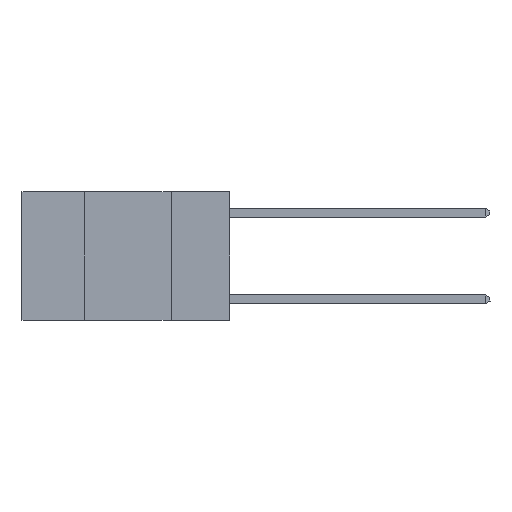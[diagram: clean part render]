
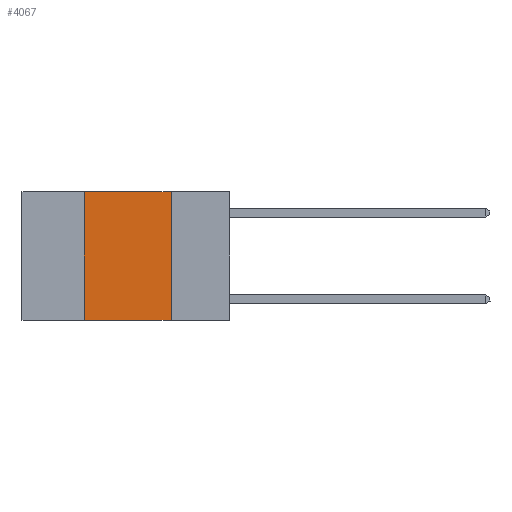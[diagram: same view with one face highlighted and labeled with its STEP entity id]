
A CAD part, left-side view. The second image highlights one B-rep face of the part: STEP entity #4067.
In plain terms, the highlighted planar face has unit normal (-1, 0, 0).
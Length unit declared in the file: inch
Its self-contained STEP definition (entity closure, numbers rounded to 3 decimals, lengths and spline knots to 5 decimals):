
#283 = DIRECTION ( 'NONE',  ( 0., 0., 1. ) ) ;
#315 = ORIENTED_EDGE ( 'NONE', *, *, #3388, .T. ) ;
#1028 = VERTEX_POINT ( 'NONE', #6104 ) ;
#1468 = EDGE_CURVE ( 'NONE', #9385, #1028, #7223, .T. ) ;
#1759 = CARTESIAN_POINT ( 'NONE',  ( 0., 0.42, 0. ) ) ;
#1832 = VECTOR ( 'NONE', #7330, 39.37008 ) ;
#2282 = VERTEX_POINT ( 'NONE', #8523 ) ;
#2452 = ORIENTED_EDGE ( 'NONE', *, *, #1468, .F. ) ;
#2545 = VERTEX_POINT ( 'NONE', #4720 ) ;
#2689 = ORIENTED_EDGE ( 'NONE', *, *, #8454, .F. ) ;
#3388 = EDGE_CURVE ( 'NONE', #2545, #2282, #8159, .T. ) ;
#3993 = DIRECTION ( 'NONE',  ( 0., 0., -1. ) ) ;
#4067 = ADVANCED_FACE ( 'NONE', ( #6612 ), #8099, .F. ) ;
#4075 = CARTESIAN_POINT ( 'NONE',  ( 0., 0.17, 0. ) ) ;
#4319 = EDGE_CURVE ( 'NONE', #1028, #2282, #6494, .T. ) ;
#4362 = CARTESIAN_POINT ( 'NONE',  ( 0., 0.6, -0.37 ) ) ;
#4720 = CARTESIAN_POINT ( 'NONE',  ( 0., 0.42, -0.37 ) ) ;
#5485 = CARTESIAN_POINT ( 'NONE',  ( 0., 0.6, 0. ) ) ;
#5611 = AXIS2_PLACEMENT_3D ( 'NONE', #8065, #8054, #8043 ) ;
#6104 = CARTESIAN_POINT ( 'NONE',  ( 0., 0.17, 0. ) ) ;
#6111 = LINE ( 'NONE', #1759, #9449 ) ;
#6176 = EDGE_LOOP ( 'NONE', ( #8215, #2452, #2689, #315 ) ) ;
#6494 = LINE ( 'NONE', #4075, #8146 ) ;
#6525 = DIRECTION ( 'NONE',  ( 0., -1., 0. ) ) ;
#6612 = FACE_OUTER_BOUND ( 'NONE', #6176, .T. ) ;
#7223 = LINE ( 'NONE', #5485, #1832 ) ;
#7330 = DIRECTION ( 'NONE',  ( 0., -1., 0. ) ) ;
#7938 = VECTOR ( 'NONE', #6525, 39.37008 ) ;
#7973 = CARTESIAN_POINT ( 'NONE',  ( 0., 0.42, 0. ) ) ;
#8043 = DIRECTION ( 'NONE',  ( 0., 0., -1. ) ) ;
#8054 = DIRECTION ( 'NONE',  ( 1., 0., 0. ) ) ;
#8065 = CARTESIAN_POINT ( 'NONE',  ( 0., 0.6, 0. ) ) ;
#8099 = PLANE ( 'NONE',  #5611 ) ;
#8146 = VECTOR ( 'NONE', #3993, 39.37008 ) ;
#8159 = LINE ( 'NONE', #4362, #7938 ) ;
#8215 = ORIENTED_EDGE ( 'NONE', *, *, #4319, .F. ) ;
#8454 = EDGE_CURVE ( 'NONE', #2545, #9385, #6111, .T. ) ;
#8523 = CARTESIAN_POINT ( 'NONE',  ( 0., 0.17, -0.37 ) ) ;
#9385 = VERTEX_POINT ( 'NONE', #7973 ) ;
#9449 = VECTOR ( 'NONE', #283, 39.37008 ) ;
